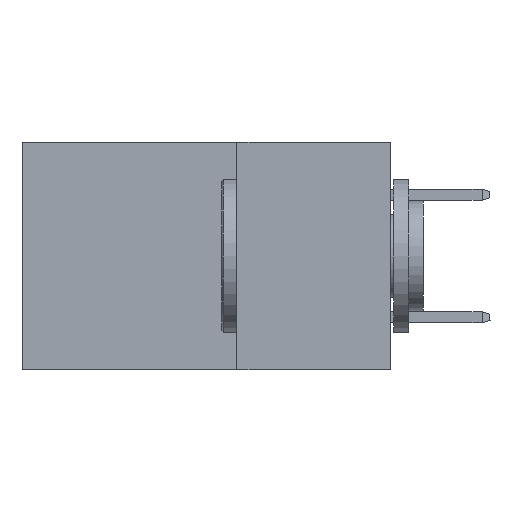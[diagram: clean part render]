
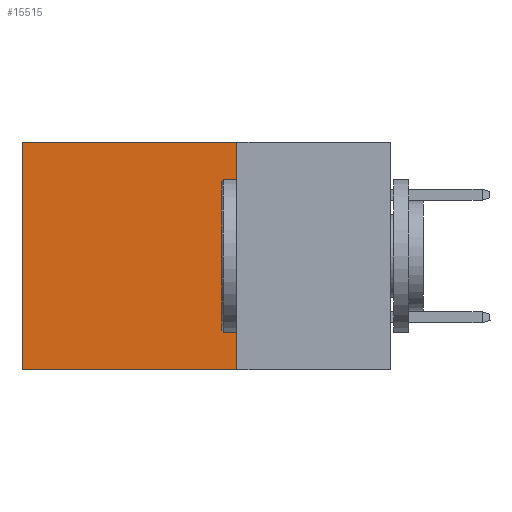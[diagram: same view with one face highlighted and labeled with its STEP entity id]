
A CAD part, left-side view. The second image highlights one B-rep face of the part: STEP entity #15515.
In plain terms, the highlighted planar face has unit normal (-1, 0, 0).
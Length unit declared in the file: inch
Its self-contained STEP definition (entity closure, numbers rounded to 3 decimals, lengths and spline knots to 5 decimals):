
#13 = PLANE ( 'NONE',  #18472 ) ;
#312 = DIRECTION ( 'NONE',  ( 0., 0., -1. ) ) ;
#442 = DIRECTION ( 'NONE',  ( 0., 1., 0. ) ) ;
#2758 = VERTEX_POINT ( 'NONE', #4599 ) ;
#3027 = DIRECTION ( 'NONE',  ( 0., 0., -1. ) ) ;
#4599 = CARTESIAN_POINT ( 'NONE',  ( 0.2875, 0.25, 0. ) ) ;
#4883 = EDGE_LOOP ( 'NONE', ( #21260, #23310, #23341, #26311 ) ) ;
#5337 = CARTESIAN_POINT ( 'NONE',  ( 0.2875, 0.25, -0.37 ) ) ;
#5379 = DIRECTION ( 'NONE',  ( 1., 0., 0. ) ) ;
#7906 = EDGE_CURVE ( 'NONE', #2758, #14880, #10663, .T. ) ;
#9145 = CARTESIAN_POINT ( 'NONE',  ( 0.2875, 0.25, 0. ) ) ;
#10663 = LINE ( 'NONE', #26424, #23484 ) ;
#14250 = DIRECTION ( 'NONE',  ( 0., 0., -1. ) ) ;
#14880 = VERTEX_POINT ( 'NONE', #26779 ) ;
#15515 = ADVANCED_FACE ( 'NONE', ( #23565 ), #13, .F. ) ;
#17153 = VECTOR ( 'NONE', #14250, 39.37008 ) ;
#17483 = VECTOR ( 'NONE', #312, 39.37008 ) ;
#17982 = CARTESIAN_POINT ( 'NONE',  ( 0.2875, 0.6, -0.37 ) ) ;
#18472 = AXIS2_PLACEMENT_3D ( 'NONE', #21116, #5379, #3027 ) ;
#19432 = EDGE_CURVE ( 'NONE', #14880, #20805, #26983, .T. ) ;
#19592 = VECTOR ( 'NONE', #29603, 39.37008 ) ;
#20805 = VERTEX_POINT ( 'NONE', #17982 ) ;
#21116 = CARTESIAN_POINT ( 'NONE',  ( 0.2875, 0.25, 0. ) ) ;
#21260 = ORIENTED_EDGE ( 'NONE', *, *, #19432, .T. ) ;
#23310 = ORIENTED_EDGE ( 'NONE', *, *, #29767, .F. ) ;
#23341 = ORIENTED_EDGE ( 'NONE', *, *, #24740, .F. ) ;
#23484 = VECTOR ( 'NONE', #442, 39.37008 ) ;
#23565 = FACE_OUTER_BOUND ( 'NONE', #4883, .T. ) ;
#23771 = LINE ( 'NONE', #5337, #19592 ) ;
#24740 = EDGE_CURVE ( 'NONE', #2758, #32263, #31674, .T. ) ;
#26311 = ORIENTED_EDGE ( 'NONE', *, *, #7906, .T. ) ;
#26424 = CARTESIAN_POINT ( 'NONE',  ( 0.2875, 0.25, 0. ) ) ;
#26779 = CARTESIAN_POINT ( 'NONE',  ( 0.2875, 0.6, 0. ) ) ;
#26983 = LINE ( 'NONE', #32224, #17483 ) ;
#29603 = DIRECTION ( 'NONE',  ( 0., 1., 0. ) ) ;
#29767 = EDGE_CURVE ( 'NONE', #32263, #20805, #23771, .T. ) ;
#30054 = CARTESIAN_POINT ( 'NONE',  ( 0.2875, 0.25, -0.37 ) ) ;
#31674 = LINE ( 'NONE', #9145, #17153 ) ;
#32224 = CARTESIAN_POINT ( 'NONE',  ( 0.2875, 0.6, 0. ) ) ;
#32263 = VERTEX_POINT ( 'NONE', #30054 ) ;
